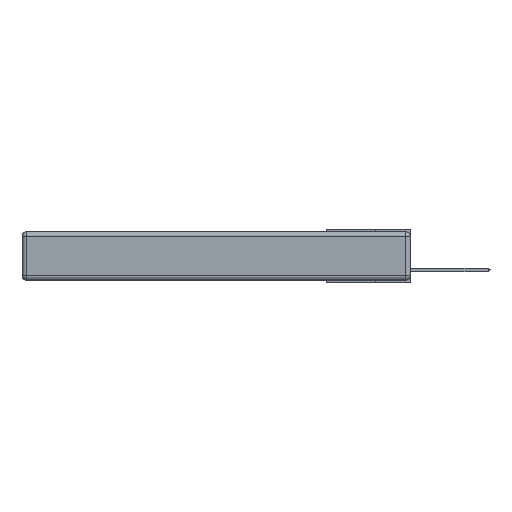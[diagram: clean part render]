
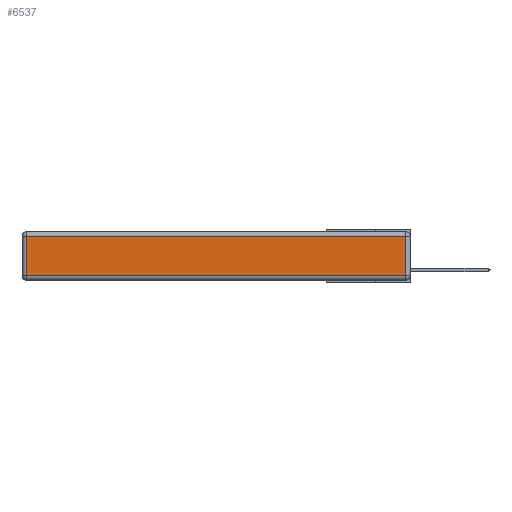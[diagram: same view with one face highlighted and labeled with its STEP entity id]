
A CAD part, left-side view. The second image highlights one B-rep face of the part: STEP entity #6537.
In plain terms, the highlighted planar face has unit normal (-1, 0, 0).
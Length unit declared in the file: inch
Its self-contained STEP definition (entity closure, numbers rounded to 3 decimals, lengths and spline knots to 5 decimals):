
#191 = VERTEX_POINT ( 'NONE', #20712 ) ;
#472 = FACE_OUTER_BOUND ( 'NONE', #20224, .T. ) ;
#1812 = CARTESIAN_POINT ( 'NONE',  ( 0., 0.03, -0.03 ) ) ;
#2480 = LINE ( 'NONE', #19427, #22761 ) ;
#3092 = EDGE_CURVE ( 'NONE', #20494, #21181, #2480, .T. ) ;
#4660 = VECTOR ( 'NONE', #13808, 39.37008 ) ;
#6537 = ADVANCED_FACE ( 'NONE', ( #472 ), #13235, .T. ) ;
#9566 = LINE ( 'NONE', #19664, #4660 ) ;
#9862 = EDGE_CURVE ( 'NONE', #191, #11439, #23809, .T. ) ;
#9964 = EDGE_CURVE ( 'NONE', #11439, #20494, #19869, .T. ) ;
#11083 = CARTESIAN_POINT ( 'NONE',  ( 0., 0., -0.343 ) ) ;
#11305 = ORIENTED_EDGE ( 'NONE', *, *, #3092, .T. ) ;
#11439 = VERTEX_POINT ( 'NONE', #1812 ) ;
#12039 = CARTESIAN_POINT ( 'NONE',  ( 0., 2.72, -0.03 ) ) ;
#12582 = ORIENTED_EDGE ( 'NONE', *, *, #18929, .T. ) ;
#13235 = PLANE ( 'NONE',  #15585 ) ;
#13808 = DIRECTION ( 'NONE',  ( 0., -1., 0. ) ) ;
#15585 = AXIS2_PLACEMENT_3D ( 'NONE', #11083, #17132, #17042 ) ;
#16140 = CARTESIAN_POINT ( 'NONE',  ( 0., 2.72, -0.313 ) ) ;
#17042 = DIRECTION ( 'NONE',  ( 0., 0., 1. ) ) ;
#17132 = DIRECTION ( 'NONE',  ( -1., 0., 0. ) ) ;
#18929 = EDGE_CURVE ( 'NONE', #21181, #191, #9566, .T. ) ;
#19183 = ORIENTED_EDGE ( 'NONE', *, *, #9964, .T. ) ;
#19427 = CARTESIAN_POINT ( 'NONE',  ( 0., 2.72, -0.343 ) ) ;
#19664 = CARTESIAN_POINT ( 'NONE',  ( 0., 0., -0.313 ) ) ;
#19869 = LINE ( 'NONE', #24892, #20141 ) ;
#20141 = VECTOR ( 'NONE', #25227, 39.37008 ) ;
#20224 = EDGE_LOOP ( 'NONE', ( #12582, #23741, #19183, #11305 ) ) ;
#20494 = VERTEX_POINT ( 'NONE', #12039 ) ;
#20712 = CARTESIAN_POINT ( 'NONE',  ( 0., 0.03, -0.313 ) ) ;
#20901 = DIRECTION ( 'NONE',  ( 0., 0., 1. ) ) ;
#21181 = VERTEX_POINT ( 'NONE', #16140 ) ;
#21388 = VECTOR ( 'NONE', #20901, 39.37008 ) ;
#22761 = VECTOR ( 'NONE', #25384, 39.37008 ) ;
#23741 = ORIENTED_EDGE ( 'NONE', *, *, #9862, .T. ) ;
#23809 = LINE ( 'NONE', #24298, #21388 ) ;
#24298 = CARTESIAN_POINT ( 'NONE',  ( 0., 0.03, -0.343 ) ) ;
#24892 = CARTESIAN_POINT ( 'NONE',  ( 0., 2.75, -0.03 ) ) ;
#25227 = DIRECTION ( 'NONE',  ( 0., 1., 0. ) ) ;
#25384 = DIRECTION ( 'NONE',  ( 0., 0., -1. ) ) ;
